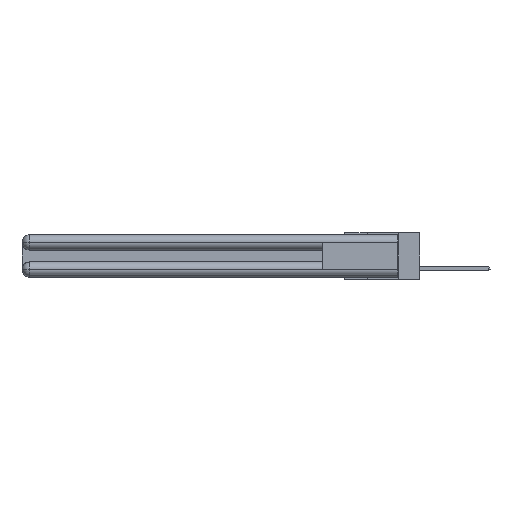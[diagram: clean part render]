
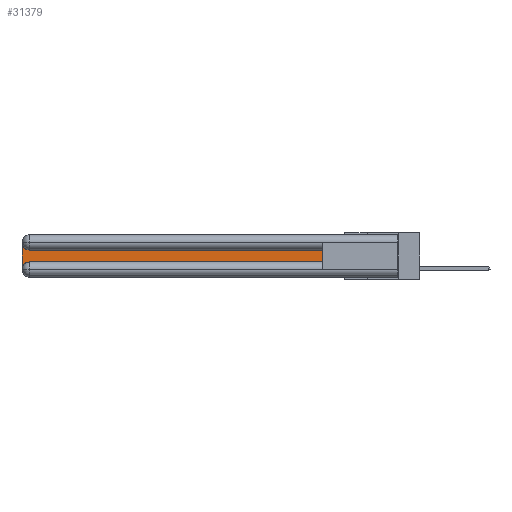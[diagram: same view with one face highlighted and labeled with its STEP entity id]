
A CAD part, left-side view. The second image highlights one B-rep face of the part: STEP entity #31379.
In plain terms, the highlighted planar face has unit normal (-1, 0, 0).
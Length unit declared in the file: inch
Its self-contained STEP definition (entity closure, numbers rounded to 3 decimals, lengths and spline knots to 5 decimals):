
#849 = PLANE ( 'NONE',  #20074 ) ;
#1087 = VERTEX_POINT ( 'NONE', #1425 ) ;
#1253 = DIRECTION ( 'NONE',  ( 0., 1., 0. ) ) ;
#1366 = ORIENTED_EDGE ( 'NONE', *, *, #20545, .T. ) ;
#1425 = CARTESIAN_POINT ( 'NONE',  ( 0.075, 0.6, -0.1225 ) ) ;
#1559 = AXIS2_PLACEMENT_3D ( 'NONE', #17717, #29949, #25491 ) ;
#2146 = EDGE_CURVE ( 'NONE', #25394, #1087, #18514, .T. ) ;
#2789 = ORIENTED_EDGE ( 'NONE', *, *, #14662, .T. ) ;
#3781 = CARTESIAN_POINT ( 'NONE',  ( 0.075, 0.6, -0.2175 ) ) ;
#4086 = LINE ( 'NONE', #29671, #16509 ) ;
#5311 = VECTOR ( 'NONE', #13020, 39.37008 ) ;
#5736 = CARTESIAN_POINT ( 'NONE',  ( 0.075, 2.94, -0.2175 ) ) ;
#7238 = VECTOR ( 'NONE', #19160, 39.37008 ) ;
#7766 = EDGE_CURVE ( 'NONE', #16789, #12989, #31148, .T. ) ;
#9169 = CARTESIAN_POINT ( 'NONE',  ( 0.075, 0.6, -0.1225 ) ) ;
#10246 = ORIENTED_EDGE ( 'NONE', *, *, #7766, .T. ) ;
#10311 = CARTESIAN_POINT ( 'NONE',  ( 0.075, 0.6, -0.2175 ) ) ;
#10921 = CARTESIAN_POINT ( 'NONE',  ( 0.075, 3., -0.1225 ) ) ;
#11769 = VERTEX_POINT ( 'NONE', #14944 ) ;
#12989 = VERTEX_POINT ( 'NONE', #29004 ) ;
#13020 = DIRECTION ( 'NONE',  ( 0., 0., 1. ) ) ;
#13267 = DIRECTION ( 'NONE',  ( 0., 0., -1. ) ) ;
#13401 = VECTOR ( 'NONE', #1253, 39.37008 ) ;
#13749 = ORIENTED_EDGE ( 'NONE', *, *, #14883, .T. ) ;
#13790 = LINE ( 'NONE', #29439, #7238 ) ;
#14662 = EDGE_CURVE ( 'NONE', #1087, #16789, #21593, .T. ) ;
#14883 = EDGE_CURVE ( 'NONE', #17427, #25394, #4086, .T. ) ;
#14944 = CARTESIAN_POINT ( 'NONE',  ( 0.075, 3., -0.2775 ) ) ;
#15091 = DIRECTION ( 'NONE',  ( 0., -1., 0. ) ) ;
#16509 = VECTOR ( 'NONE', #15091, 39.37008 ) ;
#16703 = AXIS2_PLACEMENT_3D ( 'NONE', #30545, #25215, #13267 ) ;
#16789 = VERTEX_POINT ( 'NONE', #27167 ) ;
#17427 = VERTEX_POINT ( 'NONE', #5736 ) ;
#17717 = CARTESIAN_POINT ( 'NONE',  ( 0.075, 2.94, -0.0625 ) ) ;
#17992 = FACE_OUTER_BOUND ( 'NONE', #24425, .T. ) ;
#18514 = LINE ( 'NONE', #10311, #5311 ) ;
#19160 = DIRECTION ( 'NONE',  ( 0., 0., -1. ) ) ;
#20074 = AXIS2_PLACEMENT_3D ( 'NONE', #10921, #28297, #30580 ) ;
#20545 = EDGE_CURVE ( 'NONE', #12989, #11769, #13790, .T. ) ;
#21593 = LINE ( 'NONE', #9169, #13401 ) ;
#22330 = ORIENTED_EDGE ( 'NONE', *, *, #2146, .T. ) ;
#24425 = EDGE_LOOP ( 'NONE', ( #2789, #10246, #1366, #26526, #13749, #22330 ) ) ;
#25215 = DIRECTION ( 'NONE',  ( 1., 0., 0. ) ) ;
#25394 = VERTEX_POINT ( 'NONE', #3781 ) ;
#25491 = DIRECTION ( 'NONE',  ( 0., 0., -1. ) ) ;
#26526 = ORIENTED_EDGE ( 'NONE', *, *, #27941, .T. ) ;
#27167 = CARTESIAN_POINT ( 'NONE',  ( 0.075, 2.94, -0.1225 ) ) ;
#27941 = EDGE_CURVE ( 'NONE', #11769, #17427, #28638, .T. ) ;
#28297 = DIRECTION ( 'NONE',  ( 1., 0., 0. ) ) ;
#28638 = CIRCLE ( 'NONE', #16703, 0.06 ) ;
#29004 = CARTESIAN_POINT ( 'NONE',  ( 0.075, 3., -0.0625 ) ) ;
#29439 = CARTESIAN_POINT ( 'NONE',  ( 0.075, 3., -0.2175 ) ) ;
#29671 = CARTESIAN_POINT ( 'NONE',  ( 0.075, 0.6, -0.2175 ) ) ;
#29949 = DIRECTION ( 'NONE',  ( 1., 0., 0. ) ) ;
#30545 = CARTESIAN_POINT ( 'NONE',  ( 0.075, 2.94, -0.2775 ) ) ;
#30580 = DIRECTION ( 'NONE',  ( 0., 0., -1. ) ) ;
#31148 = CIRCLE ( 'NONE', #1559, 0.06 ) ;
#31379 = ADVANCED_FACE ( 'NONE', ( #17992 ), #849, .F. ) ;
